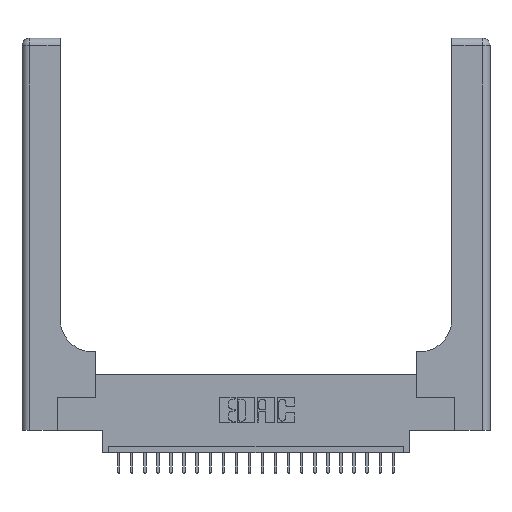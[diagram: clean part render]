
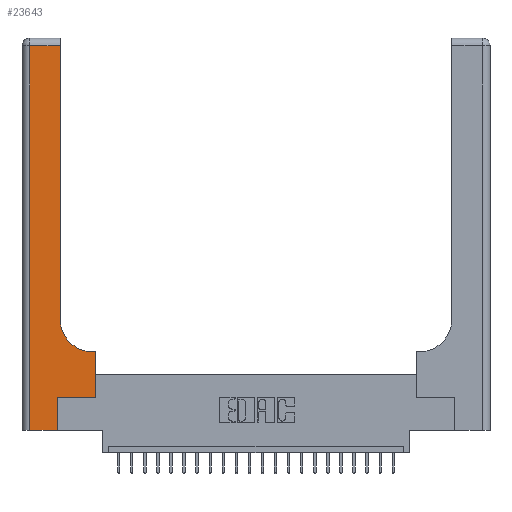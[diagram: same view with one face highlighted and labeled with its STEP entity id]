
A CAD part, top view. The second image highlights one B-rep face of the part: STEP entity #23643.
In plain terms, the highlighted planar face has unit normal (0, 0, 1).
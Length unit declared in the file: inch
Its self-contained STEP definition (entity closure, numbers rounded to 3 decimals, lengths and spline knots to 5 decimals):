
#745 = FACE_OUTER_BOUND ( 'NONE', #24369, .T. ) ;
#748 = ORIENTED_EDGE ( 'NONE', *, *, #13375, .T. ) ;
#830 = LINE ( 'NONE', #19776, #4653 ) ;
#1658 = CARTESIAN_POINT ( 'NONE',  ( 0.269, 0.25, 0.37 ) ) ;
#1898 = ORIENTED_EDGE ( 'NONE', *, *, #13446, .T. ) ;
#1900 = DIRECTION ( 'NONE',  ( -1., 0., 0. ) ) ;
#2200 = ORIENTED_EDGE ( 'NONE', *, *, #16485, .T. ) ;
#2240 = CARTESIAN_POINT ( 'NONE',  ( 0.5585, 0.6, 0.37 ) ) ;
#2414 = VECTOR ( 'NONE', #10418, 39.37008 ) ;
#3252 = VECTOR ( 'NONE', #1900, 39.37008 ) ;
#3446 = VECTOR ( 'NONE', #7101, 39.37008 ) ;
#4619 = EDGE_CURVE ( 'NONE', #21790, #16301, #19287, .T. ) ;
#4653 = VECTOR ( 'NONE', #15796, 39.37008 ) ;
#4817 = EDGE_CURVE ( 'NONE', #22425, #24006, #7141, .T. ) ;
#4821 = AXIS2_PLACEMENT_3D ( 'NONE', #19092, #21043, #17012 ) ;
#5234 = VECTOR ( 'NONE', #12168, 39.37008 ) ;
#5414 = VERTEX_POINT ( 'NONE', #5514 ) ;
#5514 = CARTESIAN_POINT ( 'NONE',  ( 0.269, 0., 0.37 ) ) ;
#5724 = CARTESIAN_POINT ( 'NONE',  ( 0.06, 0., 0.37 ) ) ;
#5806 = LINE ( 'NONE', #24492, #3446 ) ;
#6214 = ORIENTED_EDGE ( 'NONE', *, *, #4817, .T. ) ;
#6289 = CARTESIAN_POINT ( 'NONE',  ( 0.06, 3., 0.37 ) ) ;
#6300 = CARTESIAN_POINT ( 'NONE',  ( 0.5415, 0.6, 0.37 ) ) ;
#6321 = AXIS2_PLACEMENT_3D ( 'NONE', #8535, #12200, #23457 ) ;
#6343 = EDGE_CURVE ( 'NONE', #15614, #13961, #830, .T. ) ;
#6378 = CARTESIAN_POINT ( 'NONE',  ( 0., 0., 0.37 ) ) ;
#7101 = DIRECTION ( 'NONE',  ( 0., 1., 0. ) ) ;
#7141 = LINE ( 'NONE', #16907, #11558 ) ;
#8535 = CARTESIAN_POINT ( 'NONE',  ( 0.5415, 0.85, 0.37 ) ) ;
#8551 = ORIENTED_EDGE ( 'NONE', *, *, #6343, .T. ) ;
#10124 = ORIENTED_EDGE ( 'NONE', *, *, #18297, .T. ) ;
#10264 = LINE ( 'NONE', #15877, #5234 ) ;
#10418 = DIRECTION ( 'NONE',  ( 1., 0., 0. ) ) ;
#11133 = EDGE_CURVE ( 'NONE', #17364, #21790, #5806, .T. ) ;
#11198 = DIRECTION ( 'NONE',  ( 1., 0., 0. ) ) ;
#11558 = VECTOR ( 'NONE', #11198, 39.37008 ) ;
#11774 = LINE ( 'NONE', #17391, #18937 ) ;
#12091 = CIRCLE ( 'NONE', #6321, 0.25 ) ;
#12168 = DIRECTION ( 'NONE',  ( 0., 1., 0. ) ) ;
#12200 = DIRECTION ( 'NONE',  ( 0., 0., -1. ) ) ;
#12754 = ORIENTED_EDGE ( 'NONE', *, *, #4619, .T. ) ;
#13175 = PLANE ( 'NONE',  #4821 ) ;
#13254 = CARTESIAN_POINT ( 'NONE',  ( 0., 2.94, 0.37 ) ) ;
#13375 = EDGE_CURVE ( 'NONE', #16301, #14697, #18767, .T. ) ;
#13446 = EDGE_CURVE ( 'NONE', #14697, #5414, #19983, .T. ) ;
#13961 = VERTEX_POINT ( 'NONE', #6300 ) ;
#14697 = VERTEX_POINT ( 'NONE', #5724 ) ;
#15614 = VERTEX_POINT ( 'NONE', #2240 ) ;
#15796 = DIRECTION ( 'NONE',  ( -1., 0., 0. ) ) ;
#15877 = CARTESIAN_POINT ( 'NONE',  ( 0.5585, 0.25, 0.37 ) ) ;
#16218 = EDGE_CURVE ( 'NONE', #13961, #17364, #12091, .T. ) ;
#16301 = VERTEX_POINT ( 'NONE', #21567 ) ;
#16485 = EDGE_CURVE ( 'NONE', #5414, #22425, #11774, .T. ) ;
#16907 = CARTESIAN_POINT ( 'NONE',  ( 0.269, 0.25, 0.37 ) ) ;
#17012 = DIRECTION ( 'NONE',  ( -1., 0., 0. ) ) ;
#17364 = VERTEX_POINT ( 'NONE', #21959 ) ;
#17391 = CARTESIAN_POINT ( 'NONE',  ( 0.269, 0., 0.37 ) ) ;
#18297 = EDGE_CURVE ( 'NONE', #24006, #15614, #10264, .T. ) ;
#18459 = ORIENTED_EDGE ( 'NONE', *, *, #11133, .T. ) ;
#18767 = LINE ( 'NONE', #6289, #19364 ) ;
#18937 = VECTOR ( 'NONE', #23242, 39.37008 ) ;
#19092 = CARTESIAN_POINT ( 'NONE',  ( 0., 3., 0.37 ) ) ;
#19287 = LINE ( 'NONE', #13254, #3252 ) ;
#19351 = DIRECTION ( 'NONE',  ( 0., -1., 0. ) ) ;
#19364 = VECTOR ( 'NONE', #19351, 39.37008 ) ;
#19776 = CARTESIAN_POINT ( 'NONE',  ( 0.2915, 0.6, 0.37 ) ) ;
#19983 = LINE ( 'NONE', #6378, #2414 ) ;
#21043 = DIRECTION ( 'NONE',  ( 0., 0., -1. ) ) ;
#21567 = CARTESIAN_POINT ( 'NONE',  ( 0.06, 2.94, 0.37 ) ) ;
#21790 = VERTEX_POINT ( 'NONE', #24129 ) ;
#21959 = CARTESIAN_POINT ( 'NONE',  ( 0.2915, 0.85, 0.37 ) ) ;
#22425 = VERTEX_POINT ( 'NONE', #1658 ) ;
#22870 = CARTESIAN_POINT ( 'NONE',  ( 0.5585, 0.25, 0.37 ) ) ;
#23242 = DIRECTION ( 'NONE',  ( 0., 1., 0. ) ) ;
#23344 = ORIENTED_EDGE ( 'NONE', *, *, #16218, .T. ) ;
#23457 = DIRECTION ( 'NONE',  ( 1., 0., 0. ) ) ;
#23643 = ADVANCED_FACE ( 'NONE', ( #745 ), #13175, .F. ) ;
#24006 = VERTEX_POINT ( 'NONE', #22870 ) ;
#24129 = CARTESIAN_POINT ( 'NONE',  ( 0.2915, 2.94, 0.37 ) ) ;
#24369 = EDGE_LOOP ( 'NONE', ( #18459, #12754, #748, #1898, #2200, #6214, #10124, #8551, #23344 ) ) ;
#24492 = CARTESIAN_POINT ( 'NONE',  ( 0.2915, 3., 0.37 ) ) ;
